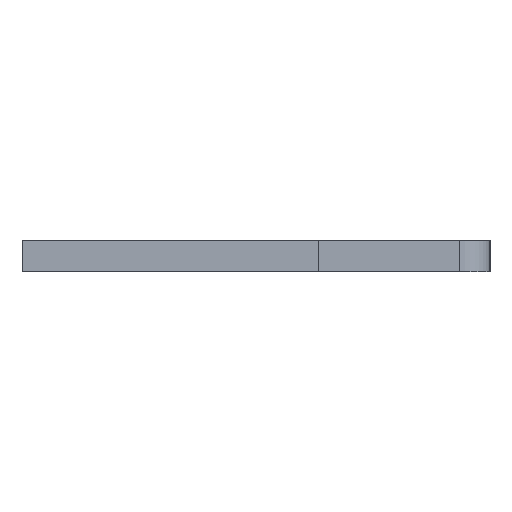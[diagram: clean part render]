
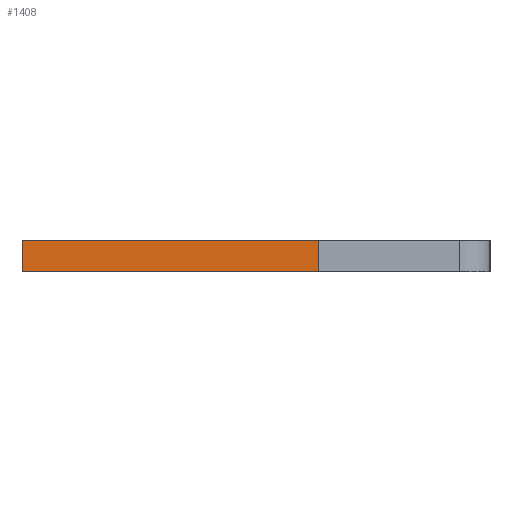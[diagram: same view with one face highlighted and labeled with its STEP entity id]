
A CAD part, left-side view. The second image highlights one B-rep face of the part: STEP entity #1408.
In plain terms, the highlighted face is planar.
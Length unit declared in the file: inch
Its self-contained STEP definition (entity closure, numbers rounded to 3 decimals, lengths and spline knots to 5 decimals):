
#21 = DIRECTION ( 'NONE',  ( 0., 0., 1. ) ) ;
#30 = DIRECTION ( 'NONE',  ( -1., 0., 0. ) ) ;
#45 = VERTEX_POINT ( 'NONE', #969 ) ;
#225 = DIRECTION ( 'NONE',  ( -1., 0., 0. ) ) ;
#235 = VECTOR ( 'NONE', #853, 39.37008 ) ;
#238 = VECTOR ( 'NONE', #1650, 39.37008 ) ;
#379 = CARTESIAN_POINT ( 'NONE',  ( 0.01, -0.04, -0.04 ) ) ;
#664 = LINE ( 'NONE', #1842, #1292 ) ;
#710 = EDGE_LOOP ( 'NONE', ( #1282, #2350, #1191, #1438 ) ) ;
#796 = PLANE ( 'NONE',  #2155 ) ;
#853 = DIRECTION ( 'NONE',  ( 0., 1., 0. ) ) ;
#907 = FACE_OUTER_BOUND ( 'NONE', #710, .T. ) ;
#969 = CARTESIAN_POINT ( 'NONE',  ( -0.01, 0.15, -0.04 ) ) ;
#1034 = CARTESIAN_POINT ( 'NONE',  ( 0.01, 0.15, -0.04 ) ) ;
#1081 = CARTESIAN_POINT ( 'NONE',  ( 0.01, -0.04, -0.04 ) ) ;
#1191 = ORIENTED_EDGE ( 'NONE', *, *, #1486, .F. ) ;
#1232 = VECTOR ( 'NONE', #30, 39.37008 ) ;
#1255 = DIRECTION ( 'NONE',  ( 1., 0., 0. ) ) ;
#1280 = CARTESIAN_POINT ( 'NONE',  ( -0.01, 0.15, -0.04 ) ) ;
#1282 = ORIENTED_EDGE ( 'NONE', *, *, #2501, .T. ) ;
#1292 = VECTOR ( 'NONE', #225, 39.37008 ) ;
#1313 = EDGE_CURVE ( 'NONE', #1830, #45, #664, .T. ) ;
#1408 = ADVANCED_FACE ( 'NONE', ( #907 ), #796, .F. ) ;
#1438 = ORIENTED_EDGE ( 'NONE', *, *, #2175, .T. ) ;
#1486 = EDGE_CURVE ( 'NONE', #1725, #1830, #1945, .T. ) ;
#1635 = VERTEX_POINT ( 'NONE', #2473 ) ;
#1644 = LINE ( 'NONE', #1280, #235 ) ;
#1650 = DIRECTION ( 'NONE',  ( 0., 1., 0. ) ) ;
#1725 = VERTEX_POINT ( 'NONE', #1081 ) ;
#1830 = VERTEX_POINT ( 'NONE', #2363 ) ;
#1842 = CARTESIAN_POINT ( 'NONE',  ( 0.01, 0.15, -0.04 ) ) ;
#1945 = LINE ( 'NONE', #1034, #238 ) ;
#2155 = AXIS2_PLACEMENT_3D ( 'NONE', #2442, #21, #1255 ) ;
#2175 = EDGE_CURVE ( 'NONE', #1725, #1635, #2422, .T. ) ;
#2350 = ORIENTED_EDGE ( 'NONE', *, *, #1313, .F. ) ;
#2363 = CARTESIAN_POINT ( 'NONE',  ( 0.01, 0.15, -0.04 ) ) ;
#2422 = LINE ( 'NONE', #379, #1232 ) ;
#2442 = CARTESIAN_POINT ( 'NONE',  ( 0.01, 0.15, -0.04 ) ) ;
#2473 = CARTESIAN_POINT ( 'NONE',  ( -0.01, -0.04, -0.04 ) ) ;
#2501 = EDGE_CURVE ( 'NONE', #1635, #45, #1644, .T. ) ;
